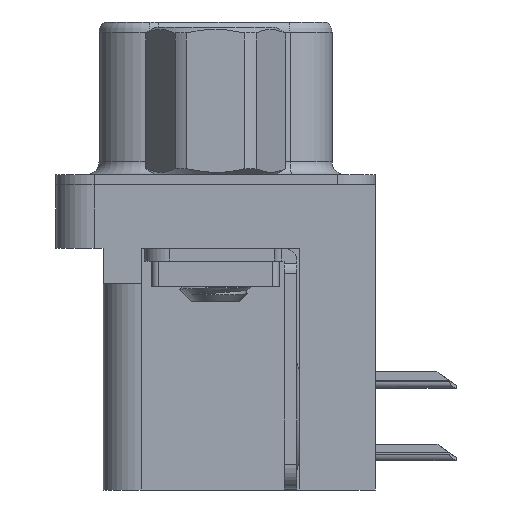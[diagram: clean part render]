
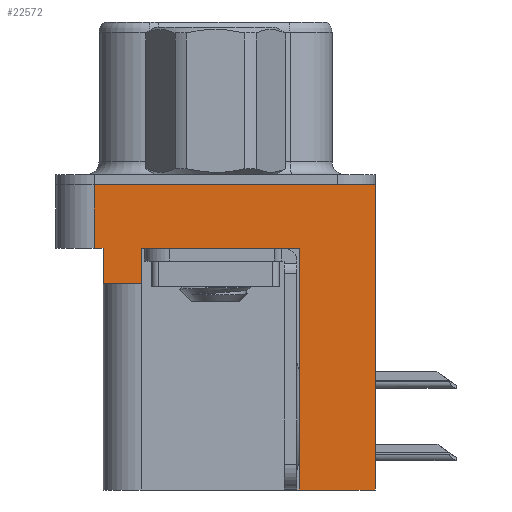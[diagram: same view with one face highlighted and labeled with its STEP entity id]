
A CAD part, left-side view. The second image highlights one B-rep face of the part: STEP entity #22572.
In plain terms, the highlighted planar face has unit normal (-1, 0, 0).
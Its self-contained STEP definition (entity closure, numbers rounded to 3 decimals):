
#70 = LINE ( 'NONE', #281, #17629 ) ;
#255 = AXIS2_PLACEMENT_3D ( 'NONE', #29441, #15940, #6728 ) ;
#280 = VECTOR ( 'NONE', #8984, 1000. ) ;
#281 = CARTESIAN_POINT ( 'NONE',  ( -3., -6.275, -2.5 ) ) ;
#288 = VERTEX_POINT ( 'NONE', #8595 ) ;
#1706 = CARTESIAN_POINT ( 'NONE',  ( -3., 4.425, -3.9 ) ) ;
#1903 = ORIENTED_EDGE ( 'NONE', *, *, #16383, .F. ) ;
#2348 = EDGE_CURVE ( 'NONE', #28316, #26289, #10673, .T. ) ;
#3062 = LINE ( 'NONE', #15082, #26648 ) ;
#4182 = DIRECTION ( 'NONE',  ( 0., -1., 0. ) ) ;
#4236 = PLANE ( 'NONE',  #255 ) ;
#4573 = CARTESIAN_POINT ( 'NONE',  ( -3., -6.275, -2.5 ) ) ;
#4690 = ORIENTED_EDGE ( 'NONE', *, *, #19399, .T. ) ;
#5412 = CARTESIAN_POINT ( 'NONE',  ( -3., 4.775, -2.5 ) ) ;
#5455 = ORIENTED_EDGE ( 'NONE', *, *, #17908, .T. ) ;
#5772 = CARTESIAN_POINT ( 'NONE',  ( -3., -6.275, -12. ) ) ;
#6088 = DIRECTION ( 'NONE',  ( 0., 0., 1. ) ) ;
#6260 = EDGE_CURVE ( 'NONE', #15565, #14245, #27736, .T. ) ;
#6352 = DIRECTION ( 'NONE',  ( 0., 1., 0. ) ) ;
#6397 = DIRECTION ( 'NONE',  ( 0., 1., 0. ) ) ;
#6420 = LINE ( 'NONE', #4573, #280 ) ;
#6715 = LINE ( 'NONE', #19856, #28448 ) ;
#6728 = DIRECTION ( 'NONE',  ( 0., 0., 1. ) ) ;
#7315 = LINE ( 'NONE', #23306, #21534 ) ;
#7876 = CARTESIAN_POINT ( 'NONE',  ( -3., 2.895, -3.9 ) ) ;
#8595 = CARTESIAN_POINT ( 'NONE',  ( -3., 2.895, -2.5 ) ) ;
#8984 = DIRECTION ( 'NONE',  ( 0., 0., 1. ) ) ;
#9691 = DIRECTION ( 'NONE',  ( 0., -1., 0. ) ) ;
#9960 = CARTESIAN_POINT ( 'NONE',  ( -3., 4.425, -2.5 ) ) ;
#10142 = ORIENTED_EDGE ( 'NONE', *, *, #2348, .F. ) ;
#10673 = LINE ( 'NONE', #1706, #22751 ) ;
#10860 = CARTESIAN_POINT ( 'NONE',  ( -3., 4.775, -2.5 ) ) ;
#11241 = VERTEX_POINT ( 'NONE', #28953 ) ;
#11622 = CARTESIAN_POINT ( 'NONE',  ( -3., -3.295, -12. ) ) ;
#11761 = DIRECTION ( 'NONE',  ( 0., 0., 1. ) ) ;
#12517 = VECTOR ( 'NONE', #21640, 1000. ) ;
#12605 = FACE_OUTER_BOUND ( 'NONE', #25879, .T. ) ;
#13542 = EDGE_CURVE ( 'NONE', #288, #20701, #7315, .T. ) ;
#14245 = VERTEX_POINT ( 'NONE', #11622 ) ;
#14510 = VERTEX_POINT ( 'NONE', #9960 ) ;
#15082 = CARTESIAN_POINT ( 'NONE',  ( -3., 4.425, -3.9 ) ) ;
#15565 = VERTEX_POINT ( 'NONE', #5772 ) ;
#15834 = CARTESIAN_POINT ( 'NONE',  ( -3., 4.425, -3.9 ) ) ;
#15940 = DIRECTION ( 'NONE',  ( -1., 0., 0. ) ) ;
#16062 = VECTOR ( 'NONE', #11761, 1000. ) ;
#16383 = EDGE_CURVE ( 'NONE', #23289, #11241, #6715, .T. ) ;
#16551 = CARTESIAN_POINT ( 'NONE',  ( -3., -3.295, -12. ) ) ;
#17232 = ORIENTED_EDGE ( 'NONE', *, *, #13542, .T. ) ;
#17629 = VECTOR ( 'NONE', #22962, 1000. ) ;
#17908 = EDGE_CURVE ( 'NONE', #27595, #14510, #70, .T. ) ;
#18286 = LINE ( 'NONE', #10860, #24350 ) ;
#18967 = EDGE_CURVE ( 'NONE', #27595, #23289, #18286, .T. ) ;
#19204 = CARTESIAN_POINT ( 'NONE',  ( -3., 2.895, -3.9 ) ) ;
#19399 = EDGE_CURVE ( 'NONE', #28316, #288, #21800, .T. ) ;
#19553 = CARTESIAN_POINT ( 'NONE',  ( -3., 4.775, 0. ) ) ;
#19856 = CARTESIAN_POINT ( 'NONE',  ( -3., -6.275, 0. ) ) ;
#20273 = EDGE_CURVE ( 'NONE', #26289, #14510, #3062, .T. ) ;
#20701 = VERTEX_POINT ( 'NONE', #23279 ) ;
#20857 = ORIENTED_EDGE ( 'NONE', *, *, #18967, .F. ) ;
#20920 = CARTESIAN_POINT ( 'NONE',  ( -3., -3.295, -12. ) ) ;
#21372 = ORIENTED_EDGE ( 'NONE', *, *, #6260, .F. ) ;
#21534 = VECTOR ( 'NONE', #9691, 1000. ) ;
#21640 = DIRECTION ( 'NONE',  ( 0., 0., 1. ) ) ;
#21800 = LINE ( 'NONE', #19204, #12517 ) ;
#22572 = ADVANCED_FACE ( 'NONE', ( #12605 ), #4236, .T. ) ;
#22751 = VECTOR ( 'NONE', #6397, 1000. ) ;
#22962 = DIRECTION ( 'NONE',  ( 0., -1., 0. ) ) ;
#23095 = VECTOR ( 'NONE', #6352, 1000. ) ;
#23279 = CARTESIAN_POINT ( 'NONE',  ( -3., -3.295, -2.5 ) ) ;
#23289 = VERTEX_POINT ( 'NONE', #19553 ) ;
#23306 = CARTESIAN_POINT ( 'NONE',  ( -3., -6.275, -2.5 ) ) ;
#23638 = EDGE_CURVE ( 'NONE', #15565, #11241, #6420, .T. ) ;
#23751 = EDGE_CURVE ( 'NONE', #14245, #20701, #28131, .T. ) ;
#24131 = ORIENTED_EDGE ( 'NONE', *, *, #20273, .F. ) ;
#24350 = VECTOR ( 'NONE', #24879, 1000. ) ;
#24879 = DIRECTION ( 'NONE',  ( 0., 0., 1. ) ) ;
#25336 = ORIENTED_EDGE ( 'NONE', *, *, #23638, .T. ) ;
#25879 = EDGE_LOOP ( 'NONE', ( #1903, #20857, #5455, #24131, #10142, #4690, #17232, #26552, #21372, #25336 ) ) ;
#26289 = VERTEX_POINT ( 'NONE', #15834 ) ;
#26552 = ORIENTED_EDGE ( 'NONE', *, *, #23751, .F. ) ;
#26648 = VECTOR ( 'NONE', #6088, 1000. ) ;
#27595 = VERTEX_POINT ( 'NONE', #5412 ) ;
#27736 = LINE ( 'NONE', #20920, #23095 ) ;
#28131 = LINE ( 'NONE', #16551, #16062 ) ;
#28316 = VERTEX_POINT ( 'NONE', #7876 ) ;
#28448 = VECTOR ( 'NONE', #4182, 1000. ) ;
#28953 = CARTESIAN_POINT ( 'NONE',  ( -3., -6.275, 0. ) ) ;
#29441 = CARTESIAN_POINT ( 'NONE',  ( -3., -6.275, -2.5 ) ) ;
